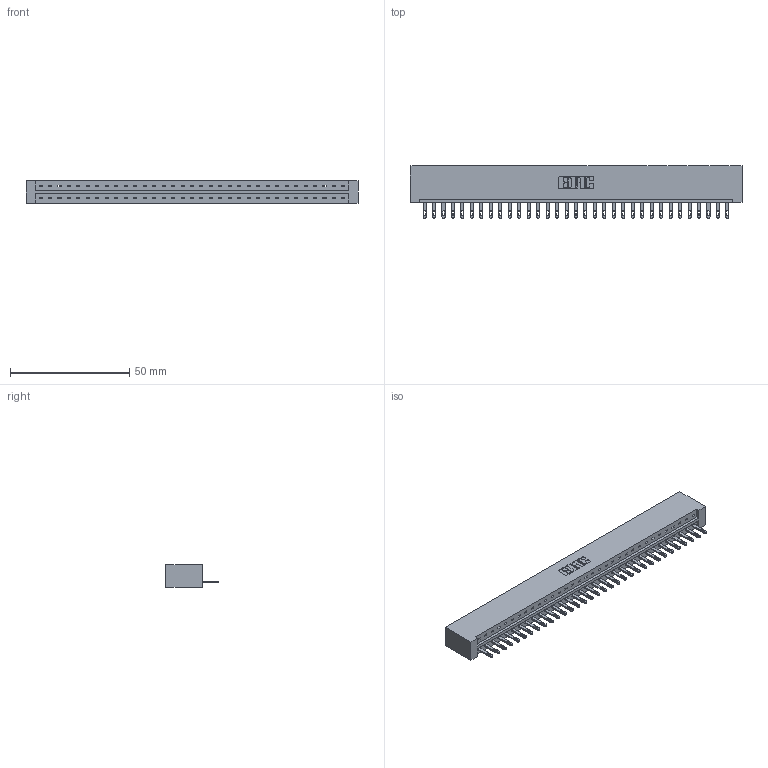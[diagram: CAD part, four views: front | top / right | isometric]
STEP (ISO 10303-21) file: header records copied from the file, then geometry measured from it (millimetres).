
FILE_DESCRIPTION (( 'STEP AP203' ), '1' );
FILE_NAME ('333-033-500-101.STEP', '2018-08-02T20:54:30', ( '' ), ( '' ), 'SwSTEP 2.0', 'SolidWorks 2016', '' );
FILE_SCHEMA (( 'CONFIG_CONTROL_DESIGN' ));
Length unit declared in the file: inch
Products named in the file (3): 333-033-500-101; 333 Part_Lugless; 345-292-001_345-293-100
Assembly tree (34 placements, depth 2):
  333-033-500-101
    333 Part_Lugless
    345-292-001_345-293-100  x33
Bounding box: 139.01 x 21.85 x 9.4 mm (x, y, z)
Volume: 14544.5 mm3; surface area: 15714.7 mm2
Topology: 34 solids, 34 shells, 1888 faces, 5831 edges, 3886 vertices
Faces by surface type: plane 1254, cylinder 634
Entity records: 20991 total; most frequent: CARTESIAN_POINT 3629, ORIENTED_EDGE 3598, DIRECTION 3073, EDGE_CURVE 1799, VECTOR 1675, LINE 1675, VERTEX_POINT 1198, AXIS2_PLACEMENT_3D 699
